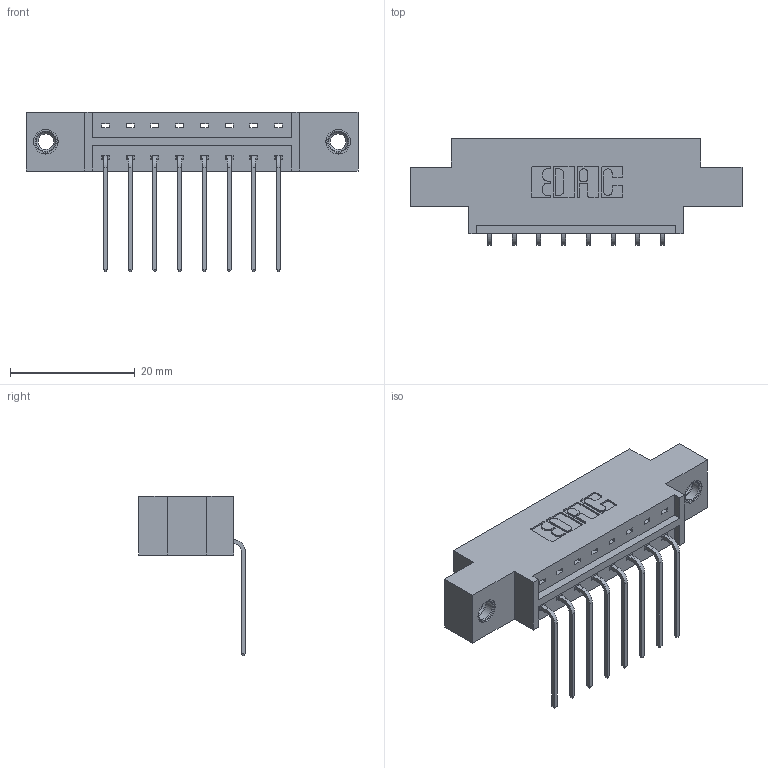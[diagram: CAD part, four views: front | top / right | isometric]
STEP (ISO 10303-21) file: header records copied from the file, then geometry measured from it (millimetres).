
FILE_DESCRIPTION (( 'STEP AP203' ), '1' );
FILE_NAME ('333-008-559-607.STEP', '2018-07-31T22:15:55', ( '' ), ( '' ), 'SwSTEP 2.0', 'SolidWorks 2016', '' );
FILE_SCHEMA (( 'CONFIG_CONTROL_DESIGN' ));
Length unit declared in the file: inch
Products named in the file (4): 333-008-559-607; 333 Part_Offset - .156 Dia - TI; 345-292-001_558 559 Tail - 1; 345-250-001_345-250-005-103
Assembly tree (11 placements, depth 2):
  333-008-559-607
    333 Part_Offset - .156 Dia - TI
    345-292-001_558 559 Tail - 1  x8
    345-250-001_345-250-005-103  x2
Bounding box: 53.24 x 17.09 x 25.53 mm (x, y, z)
Volume: 4850.2 mm3; surface area: 5424.3 mm2
Topology: 11 solids, 11 shells, 658 faces, 1915 edges, 1258 vertices
Faces by surface type: plane 458, cylinder 184, cone 12, torus 4
Entity records: 10690 total; most frequent: CARTESIAN_POINT 1833, ORIENTED_EDGE 1770, DIRECTION 1647, EDGE_CURVE 885, VECTOR 737, LINE 737, VERTEX_POINT 584, AXIS2_PLACEMENT_3D 455
